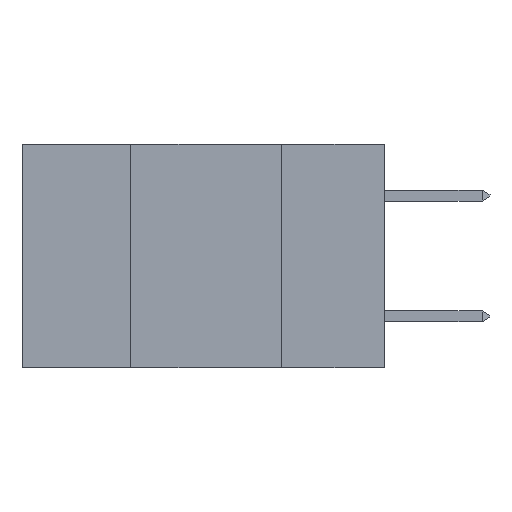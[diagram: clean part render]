
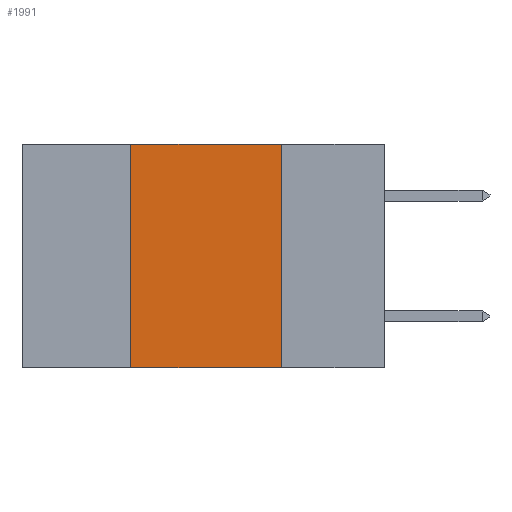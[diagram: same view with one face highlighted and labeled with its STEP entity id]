
A CAD part, left-side view. The second image highlights one B-rep face of the part: STEP entity #1991.
In plain terms, the highlighted planar face has unit normal (-1, 0, 0).
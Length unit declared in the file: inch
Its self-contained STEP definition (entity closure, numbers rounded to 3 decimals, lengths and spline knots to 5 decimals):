
#1283 = CARTESIAN_POINT ( 'NONE',  ( 0., 0.17, -0.37 ) ) ;
#1411 = VECTOR ( 'NONE', #4927, 39.37008 ) ;
#1991 = ADVANCED_FACE ( 'NONE', ( #8212 ), #8554, .F. ) ;
#3394 = LINE ( 'NONE', #16562, #9957 ) ;
#3919 = VERTEX_POINT ( 'NONE', #1283 ) ;
#4195 = EDGE_CURVE ( 'NONE', #8259, #11124, #3394, .T. ) ;
#4927 = DIRECTION ( 'NONE',  ( 0., 0., -1. ) ) ;
#5997 = LINE ( 'NONE', #10023, #1411 ) ;
#6001 = EDGE_LOOP ( 'NONE', ( #6041, #7969, #9706, #7759 ) ) ;
#6041 = ORIENTED_EDGE ( 'NONE', *, *, #12419, .F. ) ;
#6244 = AXIS2_PLACEMENT_3D ( 'NONE', #15133, #14905, #9805 ) ;
#6654 = VECTOR ( 'NONE', #13974, 39.37008 ) ;
#7205 = CARTESIAN_POINT ( 'NONE',  ( 0., 0.42, 0. ) ) ;
#7244 = EDGE_CURVE ( 'NONE', #11919, #8259, #9905, .T. ) ;
#7628 = DIRECTION ( 'NONE',  ( 0., -1., 0. ) ) ;
#7759 = ORIENTED_EDGE ( 'NONE', *, *, #14526, .T. ) ;
#7969 = ORIENTED_EDGE ( 'NONE', *, *, #4195, .F. ) ;
#8212 = FACE_OUTER_BOUND ( 'NONE', #6001, .T. ) ;
#8259 = VERTEX_POINT ( 'NONE', #9193 ) ;
#8554 = PLANE ( 'NONE',  #6244 ) ;
#8955 = VECTOR ( 'NONE', #12491, 39.37008 ) ;
#9193 = CARTESIAN_POINT ( 'NONE',  ( 0., 0.42, 0. ) ) ;
#9706 = ORIENTED_EDGE ( 'NONE', *, *, #7244, .F. ) ;
#9805 = DIRECTION ( 'NONE',  ( 0., 0., -1. ) ) ;
#9905 = LINE ( 'NONE', #7205, #6654 ) ;
#9957 = VECTOR ( 'NONE', #7628, 39.37008 ) ;
#10023 = CARTESIAN_POINT ( 'NONE',  ( 0., 0.17, 0. ) ) ;
#11124 = VERTEX_POINT ( 'NONE', #12403 ) ;
#11919 = VERTEX_POINT ( 'NONE', #13461 ) ;
#12403 = CARTESIAN_POINT ( 'NONE',  ( 0., 0.17, 0. ) ) ;
#12419 = EDGE_CURVE ( 'NONE', #11124, #3919, #5997, .T. ) ;
#12491 = DIRECTION ( 'NONE',  ( 0., -1., 0. ) ) ;
#13461 = CARTESIAN_POINT ( 'NONE',  ( 0., 0.42, -0.37 ) ) ;
#13974 = DIRECTION ( 'NONE',  ( 0., 0., 1. ) ) ;
#14526 = EDGE_CURVE ( 'NONE', #11919, #3919, #15954, .T. ) ;
#14905 = DIRECTION ( 'NONE',  ( 1., 0., 0. ) ) ;
#15103 = CARTESIAN_POINT ( 'NONE',  ( 0., 0.6, -0.37 ) ) ;
#15133 = CARTESIAN_POINT ( 'NONE',  ( 0., 0.6, 0. ) ) ;
#15954 = LINE ( 'NONE', #15103, #8955 ) ;
#16562 = CARTESIAN_POINT ( 'NONE',  ( 0., 0.6, 0. ) ) ;
